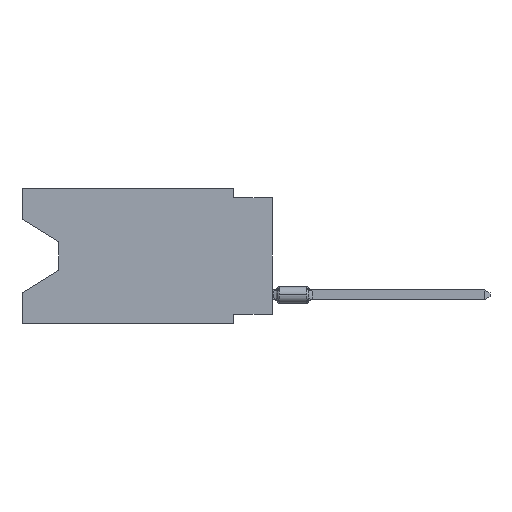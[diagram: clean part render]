
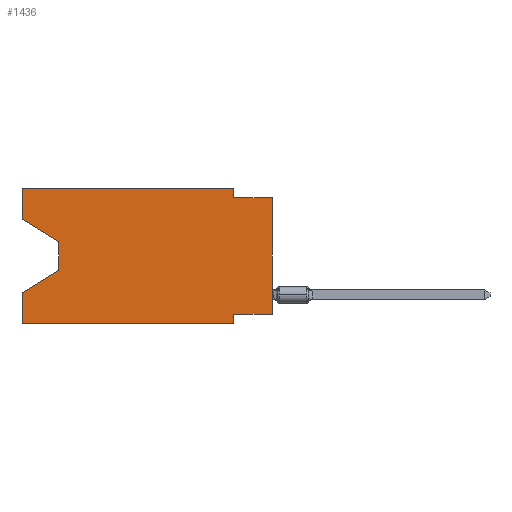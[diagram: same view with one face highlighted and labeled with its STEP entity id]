
A CAD part, left-side view. The second image highlights one B-rep face of the part: STEP entity #1436.
In plain terms, the highlighted planar face has unit normal (-1, 0, 0).
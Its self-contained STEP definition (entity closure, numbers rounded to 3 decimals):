
#111 = EDGE_CURVE ( 'NONE', #14500, #10820, #9923, .T. ) ;
#342 = ORIENTED_EDGE ( 'NONE', *, *, #6621, .F. ) ;
#924 = DIRECTION ( 'NONE',  ( 0., 0., -1. ) ) ;
#941 = VERTEX_POINT ( 'NONE', #11066 ) ;
#1027 = CARTESIAN_POINT ( 'NONE',  ( 0., 0., -8.255 ) ) ;
#1130 = CARTESIAN_POINT ( 'NONE',  ( 0., 2.54, -0.635 ) ) ;
#1436 = ADVANCED_FACE ( 'NONE', ( #6434 ), #10471, .F. ) ;
#1526 = VERTEX_POINT ( 'NONE', #7065 ) ;
#1655 = VECTOR ( 'NONE', #16230, 1000. ) ;
#1923 = CARTESIAN_POINT ( 'NONE',  ( 0., 2.54, 0. ) ) ;
#1927 = AXIS2_PLACEMENT_3D ( 'NONE', #12115, #16070, #924 ) ;
#2006 = EDGE_CURVE ( 'NONE', #8227, #10257, #16994, .T. ) ;
#2037 = CARTESIAN_POINT ( 'NONE',  ( 0., 2.54, -8.89 ) ) ;
#2322 = ORIENTED_EDGE ( 'NONE', *, *, #13849, .T. ) ;
#2629 = DIRECTION ( 'NONE',  ( 0., 0., 1. ) ) ;
#2647 = CARTESIAN_POINT ( 'NONE',  ( 0., 16.383, -8.89 ) ) ;
#2902 = ORIENTED_EDGE ( 'NONE', *, *, #9406, .T. ) ;
#3027 = VECTOR ( 'NONE', #12147, 1000. ) ;
#3327 = DIRECTION ( 'NONE',  ( 0., -1., 0. ) ) ;
#3344 = EDGE_CURVE ( 'NONE', #4644, #7134, #15897, .T. ) ;
#3443 = LINE ( 'NONE', #9404, #3027 ) ;
#3660 = VECTOR ( 'NONE', #14315, 1000. ) ;
#3715 = VECTOR ( 'NONE', #8730, 1000. ) ;
#4120 = CARTESIAN_POINT ( 'NONE',  ( 0., 16.383, 0. ) ) ;
#4397 = CARTESIAN_POINT ( 'NONE',  ( 0., 16.383, -8.89 ) ) ;
#4597 = CARTESIAN_POINT ( 'NONE',  ( 0., 13.97, -3.505 ) ) ;
#4644 = VERTEX_POINT ( 'NONE', #1130 ) ;
#5241 = VERTEX_POINT ( 'NONE', #10794 ) ;
#5603 = DIRECTION ( 'NONE',  ( 0., 1., 0. ) ) ;
#5752 = VECTOR ( 'NONE', #2629, 1000. ) ;
#5791 = EDGE_LOOP ( 'NONE', ( #17507, #17942, #2902, #342, #15033, #14041, #8560, #2322, #14425, #15633, #10714, #6356 ) ) ;
#5884 = LINE ( 'NONE', #2037, #8688 ) ;
#6169 = CARTESIAN_POINT ( 'NONE',  ( 0., 13.97, -5.385 ) ) ;
#6356 = ORIENTED_EDGE ( 'NONE', *, *, #2006, .F. ) ;
#6434 = FACE_OUTER_BOUND ( 'NONE', #5791, .T. ) ;
#6621 = EDGE_CURVE ( 'NONE', #9659, #941, #3443, .T. ) ;
#7065 = CARTESIAN_POINT ( 'NONE',  ( 0., 13.97, -5.385 ) ) ;
#7093 = DIRECTION ( 'NONE',  ( 0., -0.855, -0.519 ) ) ;
#7134 = VERTEX_POINT ( 'NONE', #16518 ) ;
#7281 = CARTESIAN_POINT ( 'NONE',  ( 0., 16.383, 0. ) ) ;
#7685 = CARTESIAN_POINT ( 'NONE',  ( 0., 16.383, 0. ) ) ;
#8227 = VERTEX_POINT ( 'NONE', #16167 ) ;
#8321 = CARTESIAN_POINT ( 'NONE',  ( 0., 2.54, -8.89 ) ) ;
#8520 = EDGE_CURVE ( 'NONE', #5241, #1526, #15684, .T. ) ;
#8560 = ORIENTED_EDGE ( 'NONE', *, *, #111, .F. ) ;
#8688 = VECTOR ( 'NONE', #13212, 1000. ) ;
#8730 = DIRECTION ( 'NONE',  ( 0., -1., 0. ) ) ;
#9404 = CARTESIAN_POINT ( 'NONE',  ( 0., 16.383, 0. ) ) ;
#9406 = EDGE_CURVE ( 'NONE', #1526, #941, #15975, .T. ) ;
#9425 = EDGE_CURVE ( 'NONE', #10820, #10007, #5884, .T. ) ;
#9659 = VERTEX_POINT ( 'NONE', #2647 ) ;
#9923 = LINE ( 'NONE', #10102, #13963 ) ;
#9997 = LINE ( 'NONE', #4120, #18062 ) ;
#10007 = VERTEX_POINT ( 'NONE', #8321 ) ;
#10102 = CARTESIAN_POINT ( 'NONE',  ( 0., 0., -8.255 ) ) ;
#10257 = VERTEX_POINT ( 'NONE', #7685 ) ;
#10471 = PLANE ( 'NONE',  #1927 ) ;
#10714 = ORIENTED_EDGE ( 'NONE', *, *, #14649, .F. ) ;
#10794 = CARTESIAN_POINT ( 'NONE',  ( 0., 13.97, -3.505 ) ) ;
#10820 = VERTEX_POINT ( 'NONE', #11368 ) ;
#10935 = EDGE_CURVE ( 'NONE', #18100, #4644, #14584, .T. ) ;
#11066 = CARTESIAN_POINT ( 'NONE',  ( 0., 16.383, -6.852 ) ) ;
#11368 = CARTESIAN_POINT ( 'NONE',  ( 0., 2.54, -8.255 ) ) ;
#12017 = CARTESIAN_POINT ( 'NONE',  ( 0., 2.54, 0. ) ) ;
#12115 = CARTESIAN_POINT ( 'NONE',  ( 0., 16.383, 0. ) ) ;
#12147 = DIRECTION ( 'NONE',  ( 0., 0., 1. ) ) ;
#12287 = EDGE_CURVE ( 'NONE', #8227, #5241, #14049, .T. ) ;
#12566 = DIRECTION ( 'NONE',  ( 0., -1., 0. ) ) ;
#12724 = VECTOR ( 'NONE', #3327, 1000. ) ;
#12852 = DIRECTION ( 'NONE',  ( 0., 0.855, -0.519 ) ) ;
#13062 = VECTOR ( 'NONE', #12852, 1000. ) ;
#13212 = DIRECTION ( 'NONE',  ( 0., 0., -1. ) ) ;
#13817 = CARTESIAN_POINT ( 'NONE',  ( 0., 0., 0. ) ) ;
#13849 = EDGE_CURVE ( 'NONE', #14500, #7134, #16669, .T. ) ;
#13963 = VECTOR ( 'NONE', #5603, 1000. ) ;
#14041 = ORIENTED_EDGE ( 'NONE', *, *, #9425, .F. ) ;
#14049 = LINE ( 'NONE', #17269, #16471 ) ;
#14315 = DIRECTION ( 'NONE',  ( 0., 0., -1. ) ) ;
#14425 = ORIENTED_EDGE ( 'NONE', *, *, #3344, .F. ) ;
#14500 = VERTEX_POINT ( 'NONE', #1027 ) ;
#14584 = LINE ( 'NONE', #1923, #15315 ) ;
#14649 = EDGE_CURVE ( 'NONE', #10257, #18100, #9997, .T. ) ;
#14721 = EDGE_CURVE ( 'NONE', #9659, #10007, #16972, .T. ) ;
#15033 = ORIENTED_EDGE ( 'NONE', *, *, #14721, .T. ) ;
#15315 = VECTOR ( 'NONE', #15665, 1000. ) ;
#15633 = ORIENTED_EDGE ( 'NONE', *, *, #10935, .F. ) ;
#15665 = DIRECTION ( 'NONE',  ( 0., 0., -1. ) ) ;
#15684 = LINE ( 'NONE', #4597, #3660 ) ;
#15897 = LINE ( 'NONE', #17280, #12724 ) ;
#15975 = LINE ( 'NONE', #6169, #13062 ) ;
#16070 = DIRECTION ( 'NONE',  ( 1., 0., 0. ) ) ;
#16167 = CARTESIAN_POINT ( 'NONE',  ( 0., 16.383, -2.038 ) ) ;
#16230 = DIRECTION ( 'NONE',  ( 0., 0., 1. ) ) ;
#16471 = VECTOR ( 'NONE', #7093, 1000. ) ;
#16518 = CARTESIAN_POINT ( 'NONE',  ( 0., 0., -0.635 ) ) ;
#16669 = LINE ( 'NONE', #13817, #5752 ) ;
#16972 = LINE ( 'NONE', #4397, #3715 ) ;
#16994 = LINE ( 'NONE', #7281, #1655 ) ;
#17269 = CARTESIAN_POINT ( 'NONE',  ( 0., 16.383, -2.038 ) ) ;
#17280 = CARTESIAN_POINT ( 'NONE',  ( 0., 0., -0.635 ) ) ;
#17507 = ORIENTED_EDGE ( 'NONE', *, *, #12287, .T. ) ;
#17942 = ORIENTED_EDGE ( 'NONE', *, *, #8520, .T. ) ;
#18062 = VECTOR ( 'NONE', #12566, 1000. ) ;
#18100 = VERTEX_POINT ( 'NONE', #12017 ) ;
